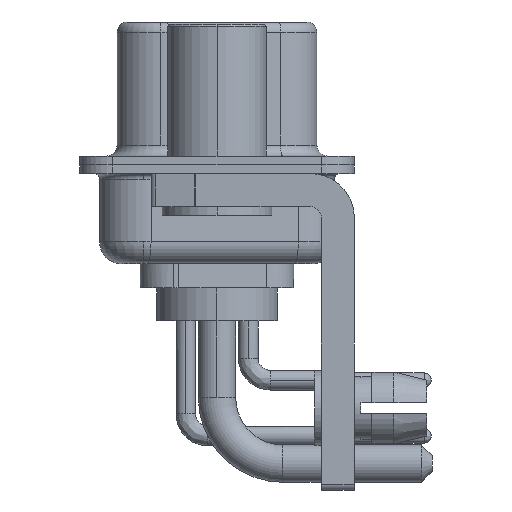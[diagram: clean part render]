
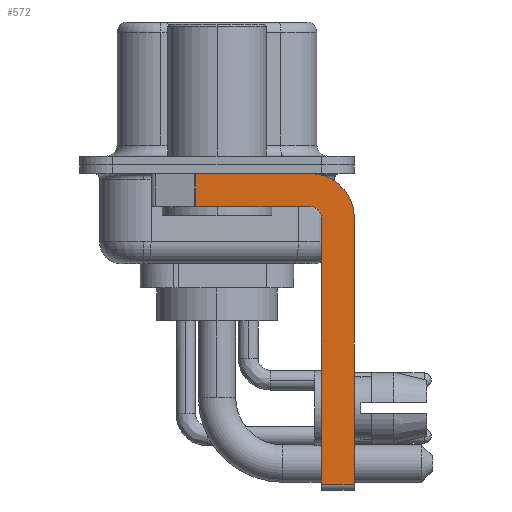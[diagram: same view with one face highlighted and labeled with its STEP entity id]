
A CAD part, left-side view. The second image highlights one B-rep face of the part: STEP entity #572.
In plain terms, the highlighted planar face has unit normal (-1, 0, 0).
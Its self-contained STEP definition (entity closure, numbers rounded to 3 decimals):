
#129 = DIRECTION ( 'NONE',  ( 0., 0., 1. ) ) ;
#572 = ADVANCED_FACE ( 'NONE', ( #18584 ), #10264, .F. ) ;
#702 = ORIENTED_EDGE ( 'NONE', *, *, #23972, .F. ) ;
#2031 = VECTOR ( 'NONE', #21405, 1000. ) ;
#2701 = CARTESIAN_POINT ( 'NONE',  ( -2.9, 0.978, -1.9 ) ) ;
#3588 = DIRECTION ( 'NONE',  ( 0., 0., -1. ) ) ;
#3660 = CARTESIAN_POINT ( 'NONE',  ( -2.9, 0.978, -1.9 ) ) ;
#4683 = EDGE_CURVE ( 'NONE', #6367, #13272, #21948, .T. ) ;
#4990 = CARTESIAN_POINT ( 'NONE',  ( -2.9, -4.75, -2.4 ) ) ;
#5692 = ORIENTED_EDGE ( 'NONE', *, *, #12588, .T. ) ;
#5903 = ORIENTED_EDGE ( 'NONE', *, *, #10610, .F. ) ;
#6367 = VERTEX_POINT ( 'NONE', #8059 ) ;
#6703 = AXIS2_PLACEMENT_3D ( 'NONE', #13228, #15114, #15246 ) ;
#7044 = CARTESIAN_POINT ( 'NONE',  ( -2.9, -4.75, -14.8 ) ) ;
#7068 = ORIENTED_EDGE ( 'NONE', *, *, #18605, .F. ) ;
#7528 = VERTEX_POINT ( 'NONE', #4990 ) ;
#7815 = DIRECTION ( 'NONE',  ( 0., -1., 0. ) ) ;
#7854 = DIRECTION ( 'NONE',  ( 0., 0., -1. ) ) ;
#8059 = CARTESIAN_POINT ( 'NONE',  ( -2.9, 0.978, -0.4 ) ) ;
#8521 = DIRECTION ( 'NONE',  ( 0., 0., -1. ) ) ;
#9830 = LINE ( 'NONE', #18013, #15324 ) ;
#10258 = VERTEX_POINT ( 'NONE', #19953 ) ;
#10264 = PLANE ( 'NONE',  #22748 ) ;
#10445 = VERTEX_POINT ( 'NONE', #20217 ) ;
#10449 = DIRECTION ( 'NONE',  ( 0., 1., 0. ) ) ;
#10610 = EDGE_CURVE ( 'NONE', #13272, #10258, #17426, .T. ) ;
#11566 = ORIENTED_EDGE ( 'NONE', *, *, #25457, .T. ) ;
#11697 = VERTEX_POINT ( 'NONE', #12707 ) ;
#12480 = CARTESIAN_POINT ( 'NONE',  ( -2.9, -4.25, -0.4 ) ) ;
#12588 = EDGE_CURVE ( 'NONE', #19599, #11697, #9830, .T. ) ;
#12707 = CARTESIAN_POINT ( 'NONE',  ( -2.9, -6.25, -14.55 ) ) ;
#13228 = CARTESIAN_POINT ( 'NONE',  ( -2.9, -4.25, -2.4 ) ) ;
#13272 = VERTEX_POINT ( 'NONE', #12480 ) ;
#14042 = CARTESIAN_POINT ( 'NONE',  ( -2.9, 3., -0.4 ) ) ;
#15114 = DIRECTION ( 'NONE',  ( 1., 0., 0. ) ) ;
#15118 = LINE ( 'NONE', #7044, #2031 ) ;
#15246 = DIRECTION ( 'NONE',  ( 0., 0., -1. ) ) ;
#15324 = VECTOR ( 'NONE', #7815, 1000. ) ;
#15547 = EDGE_CURVE ( 'NONE', #10445, #21194, #20116, .T. ) ;
#15993 = DIRECTION ( 'NONE',  ( -1., 0., 0. ) ) ;
#16227 = CARTESIAN_POINT ( 'NONE',  ( -2.9, -4.25, -1.9 ) ) ;
#16443 = DIRECTION ( 'NONE',  ( 1., 0., 0. ) ) ;
#16539 = CARTESIAN_POINT ( 'NONE',  ( -2.9, -4.25, -2.4 ) ) ;
#17426 = CIRCLE ( 'NONE', #6703, 2. ) ;
#17967 = EDGE_CURVE ( 'NONE', #10258, #11697, #17979, .T. ) ;
#17979 = LINE ( 'NONE', #20125, #21320 ) ;
#18013 = CARTESIAN_POINT ( 'NONE',  ( -2.9, -4.25, -14.55 ) ) ;
#18163 = CARTESIAN_POINT ( 'NONE',  ( -2.9, -4.75, -14.55 ) ) ;
#18501 = CIRCLE ( 'NONE', #21920, 0.5 ) ;
#18533 = ORIENTED_EDGE ( 'NONE', *, *, #15547, .F. ) ;
#18584 = FACE_OUTER_BOUND ( 'NONE', #22023, .T. ) ;
#18605 = EDGE_CURVE ( 'NONE', #19599, #7528, #15118, .T. ) ;
#19345 = VECTOR ( 'NONE', #10449, 1000. ) ;
#19599 = VERTEX_POINT ( 'NONE', #18163 ) ;
#19953 = CARTESIAN_POINT ( 'NONE',  ( -2.9, -6.25, -2.4 ) ) ;
#20116 = LINE ( 'NONE', #16227, #19345 ) ;
#20125 = CARTESIAN_POINT ( 'NONE',  ( -2.9, -6.25, -2.4 ) ) ;
#20201 = DIRECTION ( 'NONE',  ( 0., -1., 0. ) ) ;
#20217 = CARTESIAN_POINT ( 'NONE',  ( -2.9, -4.25, -1.9 ) ) ;
#21194 = VERTEX_POINT ( 'NONE', #2701 ) ;
#21320 = VECTOR ( 'NONE', #3588, 1000. ) ;
#21405 = DIRECTION ( 'NONE',  ( 0., 0., 1. ) ) ;
#21920 = AXIS2_PLACEMENT_3D ( 'NONE', #16539, #15993, #129 ) ;
#21948 = LINE ( 'NONE', #14042, #26268 ) ;
#22023 = EDGE_LOOP ( 'NONE', ( #22183, #11566, #18533, #702, #7068, #5692, #22246, #5903 ) ) ;
#22183 = ORIENTED_EDGE ( 'NONE', *, *, #4683, .F. ) ;
#22246 = ORIENTED_EDGE ( 'NONE', *, *, #17967, .F. ) ;
#22748 = AXIS2_PLACEMENT_3D ( 'NONE', #24889, #16443, #8521 ) ;
#22812 = VECTOR ( 'NONE', #7854, 1000. ) ;
#23972 = EDGE_CURVE ( 'NONE', #7528, #10445, #18501, .T. ) ;
#24889 = CARTESIAN_POINT ( 'NONE',  ( -2.9, -4.25, -2.4 ) ) ;
#25457 = EDGE_CURVE ( 'NONE', #6367, #21194, #26243, .T. ) ;
#26243 = LINE ( 'NONE', #3660, #22812 ) ;
#26268 = VECTOR ( 'NONE', #20201, 1000. ) ;
